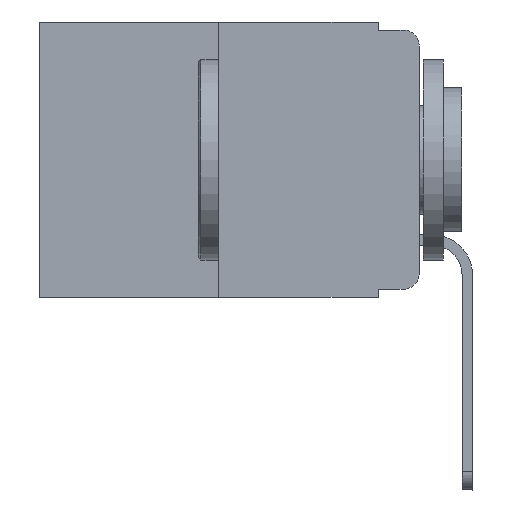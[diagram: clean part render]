
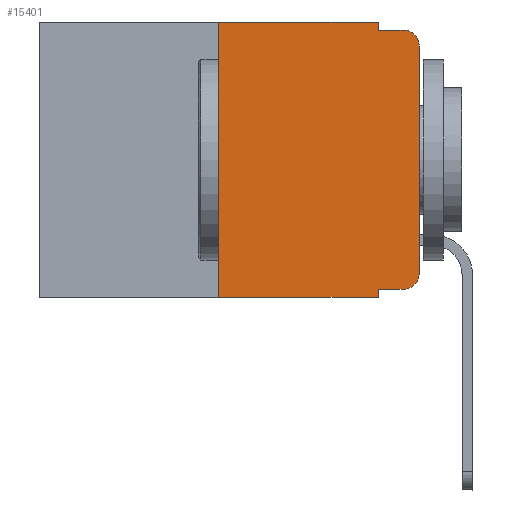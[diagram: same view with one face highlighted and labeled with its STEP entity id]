
A CAD part, left-side view. The second image highlights one B-rep face of the part: STEP entity #15401.
In plain terms, the highlighted planar face has unit normal (-1, 0, 0).
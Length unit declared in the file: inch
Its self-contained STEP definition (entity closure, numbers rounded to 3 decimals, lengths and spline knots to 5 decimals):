
#212 = VERTEX_POINT ( 'NONE', #14021 ) ;
#324 = CARTESIAN_POINT ( 'NONE',  ( 0., 0.02, -0.313 ) ) ;
#541 = EDGE_CURVE ( 'NONE', #8967, #4311, #11574, .T. ) ;
#872 = VECTOR ( 'NONE', #8237, 39.37008 ) ;
#1898 = LINE ( 'NONE', #2284, #6985 ) ;
#2108 = EDGE_CURVE ( 'NONE', #212, #19203, #11829, .T. ) ;
#2172 = CARTESIAN_POINT ( 'NONE',  ( 0., 0.473, -0.343 ) ) ;
#2284 = CARTESIAN_POINT ( 'NONE',  ( 0., 0.051, -0.333 ) ) ;
#2718 = CARTESIAN_POINT ( 'NONE',  ( 0., 0., -0.313 ) ) ;
#2953 = LINE ( 'NONE', #8997, #15781 ) ;
#2957 = EDGE_CURVE ( 'NONE', #4311, #212, #18858, .T. ) ;
#3019 = EDGE_CURVE ( 'NONE', #16397, #5493, #2953, .T. ) ;
#3992 = CARTESIAN_POINT ( 'NONE',  ( 0., 0.473, 0. ) ) ;
#4004 = DIRECTION ( 'NONE',  ( 0., 0., 1. ) ) ;
#4187 = CARTESIAN_POINT ( 'NONE',  ( 0., 0.051, 0. ) ) ;
#4198 = ORIENTED_EDGE ( 'NONE', *, *, #4787, .F. ) ;
#4304 = CARTESIAN_POINT ( 'NONE',  ( 0., 0.051, -0.01 ) ) ;
#4311 = VERTEX_POINT ( 'NONE', #2718 ) ;
#4787 = EDGE_CURVE ( 'NONE', #15482, #11508, #13501, .T. ) ;
#5083 = ORIENTED_EDGE ( 'NONE', *, *, #541, .T. ) ;
#5285 = DIRECTION ( 'NONE',  ( 0., 0., -1. ) ) ;
#5380 = PLANE ( 'NONE',  #13294 ) ;
#5493 = VERTEX_POINT ( 'NONE', #18859 ) ;
#5698 = LINE ( 'NONE', #13238, #15822 ) ;
#5705 = DIRECTION ( 'NONE',  ( 0., 0., 1. ) ) ;
#6007 = CARTESIAN_POINT ( 'NONE',  ( 0., 0.051, -0.343 ) ) ;
#6473 = CARTESIAN_POINT ( 'NONE',  ( 0., 0.25, 0. ) ) ;
#6630 = DIRECTION ( 'NONE',  ( 0., -1., 0. ) ) ;
#6985 = VECTOR ( 'NONE', #15570, 39.37008 ) ;
#7088 = CARTESIAN_POINT ( 'NONE',  ( 0., 0.25, 0. ) ) ;
#7255 = VECTOR ( 'NONE', #5705, 39.37008 ) ;
#8237 = DIRECTION ( 'NONE',  ( 0., -1., 0. ) ) ;
#8472 = EDGE_LOOP ( 'NONE', ( #11282, #14587, #10723, #9971, #19528, #9684, #8777, #4198, #12754, #5083 ) ) ;
#8777 = ORIENTED_EDGE ( 'NONE', *, *, #10877, .T. ) ;
#8967 = VERTEX_POINT ( 'NONE', #16290 ) ;
#8997 = CARTESIAN_POINT ( 'NONE',  ( 0., 0.473, 0. ) ) ;
#9439 = DIRECTION ( 'NONE',  ( -1., 0., 0. ) ) ;
#9684 = ORIENTED_EDGE ( 'NONE', *, *, #11320, .F. ) ;
#9758 = LINE ( 'NONE', #7088, #16717 ) ;
#9849 = VECTOR ( 'NONE', #10531, 39.37008 ) ;
#9971 = ORIENTED_EDGE ( 'NONE', *, *, #13772, .F. ) ;
#10177 = DIRECTION ( 'NONE',  ( 0., -1., 0. ) ) ;
#10531 = DIRECTION ( 'NONE',  ( 0., 0., -1. ) ) ;
#10723 = ORIENTED_EDGE ( 'NONE', *, *, #13070, .F. ) ;
#10877 = EDGE_CURVE ( 'NONE', #13010, #11508, #18721, .T. ) ;
#10996 = CARTESIAN_POINT ( 'NONE',  ( 0., 0.051, -0.01 ) ) ;
#11157 = DIRECTION ( 'NONE',  ( 0., 0., -1. ) ) ;
#11282 = ORIENTED_EDGE ( 'NONE', *, *, #2957, .T. ) ;
#11320 = EDGE_CURVE ( 'NONE', #13010, #16397, #9758, .T. ) ;
#11441 = DIRECTION ( 'NONE',  ( 1., 0., 0. ) ) ;
#11508 = VERTEX_POINT ( 'NONE', #6007 ) ;
#11574 = CIRCLE ( 'NONE', #12536, 0.02 ) ;
#11603 = CARTESIAN_POINT ( 'NONE',  ( 0., 0.02, -0.03 ) ) ;
#11643 = DIRECTION ( 'NONE',  ( 0., 0., -1. ) ) ;
#11729 = VECTOR ( 'NONE', #6630, 39.37008 ) ;
#11829 = CIRCLE ( 'NONE', #14300, 0.02 ) ;
#12492 = LINE ( 'NONE', #10996, #11729 ) ;
#12536 = AXIS2_PLACEMENT_3D ( 'NONE', #324, #9439, #18536 ) ;
#12754 = ORIENTED_EDGE ( 'NONE', *, *, #16347, .T. ) ;
#13010 = VERTEX_POINT ( 'NONE', #14964 ) ;
#13070 = EDGE_CURVE ( 'NONE', #15551, #19203, #12492, .T. ) ;
#13238 = CARTESIAN_POINT ( 'NONE',  ( 0., 0.051, 0. ) ) ;
#13294 = AXIS2_PLACEMENT_3D ( 'NONE', #3992, #11441, #5285 ) ;
#13501 = LINE ( 'NONE', #4187, #9849 ) ;
#13772 = EDGE_CURVE ( 'NONE', #5493, #15551, #5698, .T. ) ;
#14021 = CARTESIAN_POINT ( 'NONE',  ( 0., 0., -0.03 ) ) ;
#14300 = AXIS2_PLACEMENT_3D ( 'NONE', #11603, #15685, #11157 ) ;
#14587 = ORIENTED_EDGE ( 'NONE', *, *, #2108, .T. ) ;
#14964 = CARTESIAN_POINT ( 'NONE',  ( 0., 0.25, -0.343 ) ) ;
#15085 = CARTESIAN_POINT ( 'NONE',  ( 0., 0.051, -0.333 ) ) ;
#15401 = ADVANCED_FACE ( 'NONE', ( #18932 ), #5380, .F. ) ;
#15482 = VERTEX_POINT ( 'NONE', #15085 ) ;
#15551 = VERTEX_POINT ( 'NONE', #4304 ) ;
#15570 = DIRECTION ( 'NONE',  ( 0., -1., 0. ) ) ;
#15685 = DIRECTION ( 'NONE',  ( -1., 0., 0. ) ) ;
#15781 = VECTOR ( 'NONE', #10177, 39.37008 ) ;
#15822 = VECTOR ( 'NONE', #11643, 39.37008 ) ;
#16290 = CARTESIAN_POINT ( 'NONE',  ( 0., 0.02, -0.333 ) ) ;
#16347 = EDGE_CURVE ( 'NONE', #15482, #8967, #1898, .T. ) ;
#16397 = VERTEX_POINT ( 'NONE', #6473 ) ;
#16520 = CARTESIAN_POINT ( 'NONE',  ( 0., 0., 0. ) ) ;
#16717 = VECTOR ( 'NONE', #4004, 39.37008 ) ;
#16744 = CARTESIAN_POINT ( 'NONE',  ( 0., 0.02, -0.01 ) ) ;
#18536 = DIRECTION ( 'NONE',  ( 0., 0., -1. ) ) ;
#18721 = LINE ( 'NONE', #2172, #872 ) ;
#18858 = LINE ( 'NONE', #16520, #7255 ) ;
#18859 = CARTESIAN_POINT ( 'NONE',  ( 0., 0.051, 0. ) ) ;
#18932 = FACE_OUTER_BOUND ( 'NONE', #8472, .T. ) ;
#19203 = VERTEX_POINT ( 'NONE', #16744 ) ;
#19528 = ORIENTED_EDGE ( 'NONE', *, *, #3019, .F. ) ;
